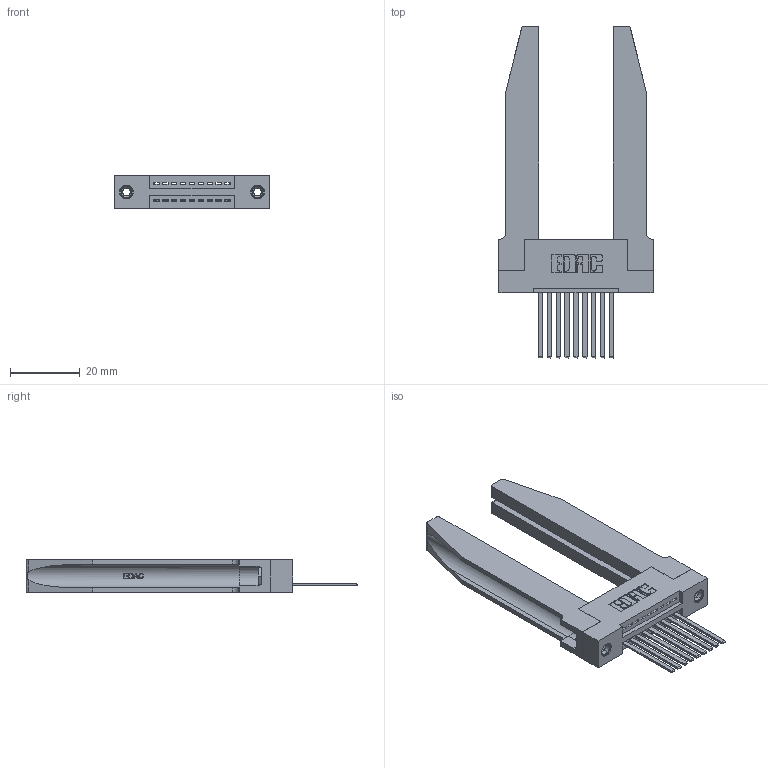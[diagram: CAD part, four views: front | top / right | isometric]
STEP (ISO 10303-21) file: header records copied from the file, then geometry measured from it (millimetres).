
FILE_DESCRIPTION (( 'STEP AP203' ), '1' );
FILE_NAME ('395-009-544-178.STEP', '2019-10-15T20:43:40', ( '' ), ( '' ), 'SwSTEP 2.0', 'SolidWorks 2016', '' );
FILE_SCHEMA (( 'CONFIG_CONTROL_DESIGN' ));
Length unit declared in the file: inch
Products named in the file (5): 345-250-001_345-250-001-102; 345-292-001_345-293-144; 345 Part_Flush Mounting Lugs - 0.156 Dia-TH; 345-220-078_345-220-078; 395-009-544-178
Assembly tree (14 placements, depth 2):
  395-009-544-178
    345 Part_Flush Mounting Lugs - 0.156 Dia-TH
    345-292-001_345-293-144  x9
    345-250-001_345-250-001-102  x2
    345-220-078_345-220-078  x2
Bounding box: 44.09 x 94.92 x 9.4 mm (x, y, z)
Volume: 11792.5 mm3; surface area: 12054.9 mm2
Topology: 14 solids, 14 shells, 828 faces, 2371 edges, 1558 vertices
Faces by surface type: plane 546, cylinder 230, bspline 36, cone 12, torus 4
Entity records: 15772 total; most frequent: CARTESIAN_POINT 3630, ORIENTED_EDGE 2470, DIRECTION 2223, EDGE_CURVE 1235, LINE 977, VECTOR 977, VERTEX_POINT 816, AXIS2_PLACEMENT_3D 623
